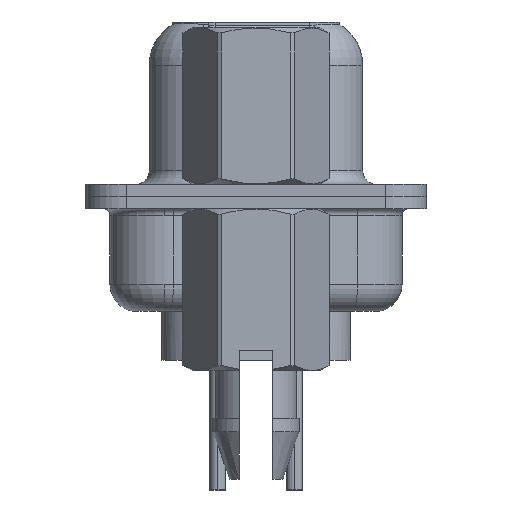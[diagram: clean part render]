
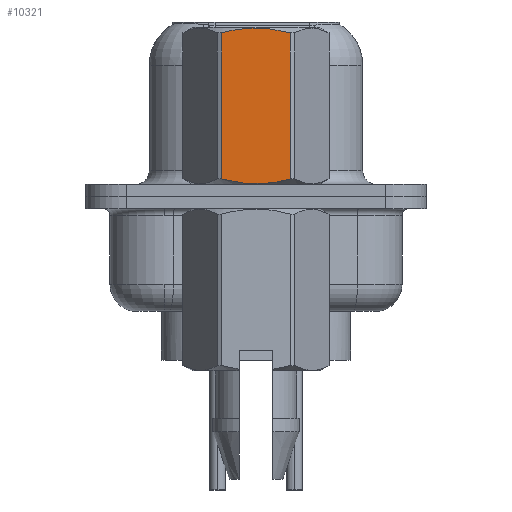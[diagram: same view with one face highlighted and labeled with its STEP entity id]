
A CAD part, left-side view. The second image highlights one B-rep face of the part: STEP entity #10321.
In plain terms, the highlighted planar face has unit normal (-1, 0, 0).
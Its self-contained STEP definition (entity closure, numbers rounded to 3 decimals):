
#121 = CARTESIAN_POINT ( 'NONE',  ( -2.381, -0.215, 0.468 ) ) ;
#1024 = CARTESIAN_POINT ( 'NONE',  ( -2.381, -1.273, 0.652 ) ) ;
#1214 = CARTESIAN_POINT ( 'NONE',  ( -2.381, 1.375, -3.75 ) ) ;
#1415 = VECTOR ( 'NONE', #5485, 1000. ) ;
#2012 = CARTESIAN_POINT ( 'NONE',  ( -2.381, 1.273, 0.652 ) ) ;
#2373 = VERTEX_POINT ( 'NONE', #1024 ) ;
#2411 = CARTESIAN_POINT ( 'NONE',  ( -2.381, 0.428, 0.485 ) ) ;
#3328 = DIRECTION ( 'NONE',  ( -1., 0., 0. ) ) ;
#3506 = LINE ( 'NONE', #7752, #1415 ) ;
#4799 = EDGE_CURVE ( 'NONE', #26515, #22288, #9349, .T. ) ;
#4879 = AXIS2_PLACEMENT_3D ( 'NONE', #1214, #3328, #17355 ) ;
#5138 = CARTESIAN_POINT ( 'NONE',  ( -2.381, 0.215, 0.468 ) ) ;
#5288 = CARTESIAN_POINT ( 'NONE',  ( -2.381, -1.066, 0.596 ) ) ;
#5485 = DIRECTION ( 'NONE',  ( 0., 0., 1. ) ) ;
#5731 = CARTESIAN_POINT ( 'NONE',  ( -2.381, -1.273, 6.048 ) ) ;
#6964 = CARTESIAN_POINT ( 'NONE',  ( -2.381, -0.432, 0.485 ) ) ;
#7752 = CARTESIAN_POINT ( 'NONE',  ( -2.381, -1.273, 3.792 ) ) ;
#8156 = CARTESIAN_POINT ( 'NONE',  ( -2.381, 0.428, 6.215 ) ) ;
#9349 = LINE ( 'NONE', #27882, #12375 ) ;
#10321 = ADVANCED_FACE ( 'NONE', ( #22057 ), #19632, .T. ) ;
#11999 = CARTESIAN_POINT ( 'NONE',  ( -2.381, 1.065, 0.596 ) ) ;
#12375 = VECTOR ( 'NONE', #16056, 1000. ) ;
#12448 = CARTESIAN_POINT ( 'NONE',  ( -2.381, -0.432, 6.215 ) ) ;
#13229 = EDGE_LOOP ( 'NONE', ( #28942, #13702, #28039, #15015 ) ) ;
#13645 = EDGE_CURVE ( 'NONE', #2373, #14188, #3506, .T. ) ;
#13702 = ORIENTED_EDGE ( 'NONE', *, *, #13645, .T. ) ;
#14041 = EDGE_CURVE ( 'NONE', #22288, #2373, #20304, .T. ) ;
#14188 = VERTEX_POINT ( 'NONE', #19917 ) ;
#15015 = ORIENTED_EDGE ( 'NONE', *, *, #4799, .T. ) ;
#15196 = CARTESIAN_POINT ( 'NONE',  ( -2.381, -0.858, 6.15 ) ) ;
#16056 = DIRECTION ( 'NONE',  ( 0., 0., -1. ) ) ;
#16729 = CARTESIAN_POINT ( 'NONE',  ( -2.381, 0.853, 0.549 ) ) ;
#17333 = CARTESIAN_POINT ( 'NONE',  ( -2.381, -0.215, 6.232 ) ) ;
#17355 = DIRECTION ( 'NONE',  ( 0., -1., 0. ) ) ;
#19029 = CARTESIAN_POINT ( 'NONE',  ( -2.381, 1.273, 6.048 ) ) ;
#19296 = CARTESIAN_POINT ( 'NONE',  ( -2.381, 0.215, 6.232 ) ) ;
#19603 = CARTESIAN_POINT ( 'NONE',  ( -2.381, 1.273, 6.048 ) ) ;
#19632 = PLANE ( 'NONE',  #4879 ) ;
#19917 = CARTESIAN_POINT ( 'NONE',  ( -2.381, -1.273, 6.048 ) ) ;
#20304 = B_SPLINE_CURVE_WITH_KNOTS ( 'NONE', 3,
 ( #28376, #11999, #16729, #2411, #5138, #121, #6964, #21430, #5288, #30045 ),
 .UNSPECIFIED., .F., .F.,
 ( 4, 2, 2, 2, 4 ),
 ( 0.003, 0.003, 0.004, 0.004, 0.005 ),
 .UNSPECIFIED. ) ;
#21430 = CARTESIAN_POINT ( 'NONE',  ( -2.381, -0.858, 0.55 ) ) ;
#22057 = FACE_OUTER_BOUND ( 'NONE', #13229, .T. ) ;
#22288 = VERTEX_POINT ( 'NONE', #2012 ) ;
#22412 = B_SPLINE_CURVE_WITH_KNOTS ( 'NONE', 3,
 ( #5731, #26427, #15196, #12448, #17333, #19296, #8156, #24286, #24451, #19603 ),
 .UNSPECIFIED., .F., .F.,
 ( 4, 2, 2, 2, 4 ),
 ( 0.001, 0.002, 0.002, 0.003, 0.004 ),
 .UNSPECIFIED. ) ;
#24286 = CARTESIAN_POINT ( 'NONE',  ( -2.381, 0.853, 6.151 ) ) ;
#24451 = CARTESIAN_POINT ( 'NONE',  ( -2.381, 1.065, 6.104 ) ) ;
#26427 = CARTESIAN_POINT ( 'NONE',  ( -2.381, -1.066, 6.104 ) ) ;
#26515 = VERTEX_POINT ( 'NONE', #19029 ) ;
#26896 = EDGE_CURVE ( 'NONE', #14188, #26515, #22412, .T. ) ;
#27882 = CARTESIAN_POINT ( 'NONE',  ( -2.381, 1.273, 3.792 ) ) ;
#28039 = ORIENTED_EDGE ( 'NONE', *, *, #26896, .T. ) ;
#28376 = CARTESIAN_POINT ( 'NONE',  ( -2.381, 1.273, 0.652 ) ) ;
#28942 = ORIENTED_EDGE ( 'NONE', *, *, #14041, .T. ) ;
#30045 = CARTESIAN_POINT ( 'NONE',  ( -2.381, -1.273, 0.652 ) ) ;
